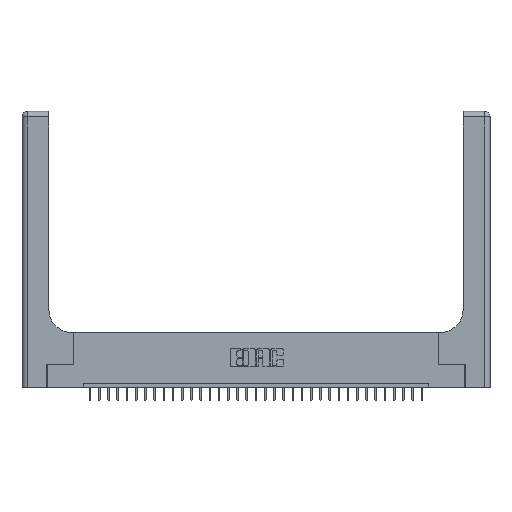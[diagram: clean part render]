
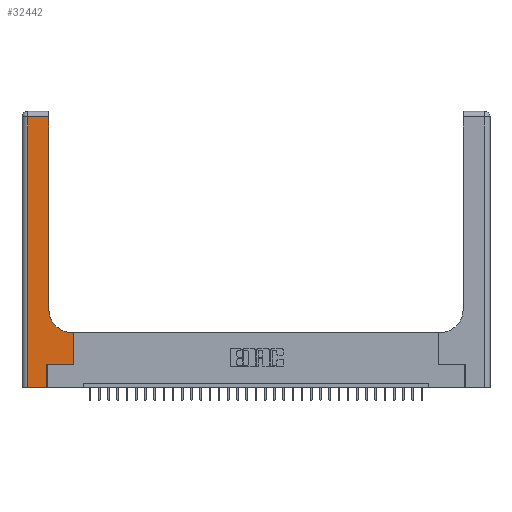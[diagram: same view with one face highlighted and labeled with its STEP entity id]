
A CAD part, top view. The second image highlights one B-rep face of the part: STEP entity #32442.
In plain terms, the highlighted planar face has unit normal (0, 0, 1).
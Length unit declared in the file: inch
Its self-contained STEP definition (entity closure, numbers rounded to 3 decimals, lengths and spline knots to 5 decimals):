
#429 = LINE ( 'NONE', #18204, #14327 ) ;
#706 = VECTOR ( 'NONE', #27612, 39.37008 ) ;
#1019 = ORIENTED_EDGE ( 'NONE', *, *, #8162, .T. ) ;
#1264 = CARTESIAN_POINT ( 'NONE',  ( 0., 3., 0.37 ) ) ;
#1698 = ORIENTED_EDGE ( 'NONE', *, *, #15949, .T. ) ;
#2231 = CARTESIAN_POINT ( 'NONE',  ( 0.2915, 2.94, 0.37 ) ) ;
#3149 = EDGE_CURVE ( 'NONE', #30729, #19124, #429, .T. ) ;
#3225 = CARTESIAN_POINT ( 'NONE',  ( 0.5585, 0.6, 0.37 ) ) ;
#3916 = VERTEX_POINT ( 'NONE', #15394 ) ;
#4030 = CARTESIAN_POINT ( 'NONE',  ( 0.5585, 0.25, 0.37 ) ) ;
#4856 = VERTEX_POINT ( 'NONE', #22774 ) ;
#4884 = VECTOR ( 'NONE', #11220, 39.37008 ) ;
#5099 = CARTESIAN_POINT ( 'NONE',  ( 0.269, 0.25, 0.37 ) ) ;
#5725 = VERTEX_POINT ( 'NONE', #14816 ) ;
#6224 = DIRECTION ( 'NONE',  ( 0., 0., -1. ) ) ;
#6456 = CARTESIAN_POINT ( 'NONE',  ( 0.269, 0.25, 0.37 ) ) ;
#6606 = AXIS2_PLACEMENT_3D ( 'NONE', #27712, #25154, #14715 ) ;
#7086 = EDGE_LOOP ( 'NONE', ( #30935, #1698, #17297, #32505, #23765, #1019, #29211, #14005, #7499 ) ) ;
#7499 = ORIENTED_EDGE ( 'NONE', *, *, #12055, .T. ) ;
#8162 = EDGE_CURVE ( 'NONE', #22408, #3916, #24742, .T. ) ;
#8231 = EDGE_CURVE ( 'NONE', #5725, #12000, #15760, .T. ) ;
#8516 = VERTEX_POINT ( 'NONE', #30452 ) ;
#8628 = AXIS2_PLACEMENT_3D ( 'NONE', #1264, #6224, #22279 ) ;
#9114 = CARTESIAN_POINT ( 'NONE',  ( 0., 0., 0.37 ) ) ;
#10355 = CARTESIAN_POINT ( 'NONE',  ( 0.269, 0., 0.37 ) ) ;
#11220 = DIRECTION ( 'NONE',  ( 1., 0., 0. ) ) ;
#12000 = VERTEX_POINT ( 'NONE', #2231 ) ;
#12055 = EDGE_CURVE ( 'NONE', #19124, #5725, #33334, .T. ) ;
#12588 = EDGE_CURVE ( 'NONE', #4856, #22408, #33799, .T. ) ;
#13820 = VECTOR ( 'NONE', #19882, 39.37008 ) ;
#13849 = CARTESIAN_POINT ( 'NONE',  ( 0.5415, 0.6, 0.37 ) ) ;
#14005 = ORIENTED_EDGE ( 'NONE', *, *, #3149, .T. ) ;
#14327 = VECTOR ( 'NONE', #21275, 39.37008 ) ;
#14525 = EDGE_CURVE ( 'NONE', #3916, #30729, #19733, .T. ) ;
#14715 = DIRECTION ( 'NONE',  ( 1., 0., 0. ) ) ;
#14816 = CARTESIAN_POINT ( 'NONE',  ( 0.2915, 0.85, 0.37 ) ) ;
#15394 = CARTESIAN_POINT ( 'NONE',  ( 0.5585, 0.25, 0.37 ) ) ;
#15760 = LINE ( 'NONE', #22509, #30517 ) ;
#15949 = EDGE_CURVE ( 'NONE', #12000, #8516, #23826, .T. ) ;
#15999 = CARTESIAN_POINT ( 'NONE',  ( 0.06, 0., 0.37 ) ) ;
#17297 = ORIENTED_EDGE ( 'NONE', *, *, #25033, .T. ) ;
#17875 = DIRECTION ( 'NONE',  ( 0., 1., 0. ) ) ;
#18204 = CARTESIAN_POINT ( 'NONE',  ( 0.2915, 0.6, 0.37 ) ) ;
#18245 = DIRECTION ( 'NONE',  ( 0., 1., 0. ) ) ;
#19029 = FACE_OUTER_BOUND ( 'NONE', #7086, .T. ) ;
#19124 = VERTEX_POINT ( 'NONE', #13849 ) ;
#19191 = CARTESIAN_POINT ( 'NONE',  ( 0., 2.94, 0.37 ) ) ;
#19733 = LINE ( 'NONE', #4030, #26926 ) ;
#19882 = DIRECTION ( 'NONE',  ( 1., 0., 0. ) ) ;
#19921 = LINE ( 'NONE', #32729, #706 ) ;
#21067 = VERTEX_POINT ( 'NONE', #15999 ) ;
#21275 = DIRECTION ( 'NONE',  ( -1., 0., 0. ) ) ;
#21936 = LINE ( 'NONE', #9114, #13820 ) ;
#22279 = DIRECTION ( 'NONE',  ( -1., 0., 0. ) ) ;
#22408 = VERTEX_POINT ( 'NONE', #5099 ) ;
#22509 = CARTESIAN_POINT ( 'NONE',  ( 0.2915, 3., 0.37 ) ) ;
#22774 = CARTESIAN_POINT ( 'NONE',  ( 0.269, 0., 0.37 ) ) ;
#23765 = ORIENTED_EDGE ( 'NONE', *, *, #12588, .T. ) ;
#23826 = LINE ( 'NONE', #19191, #32461 ) ;
#24644 = VECTOR ( 'NONE', #18245, 39.37008 ) ;
#24742 = LINE ( 'NONE', #6456, #4884 ) ;
#25033 = EDGE_CURVE ( 'NONE', #8516, #21067, #19921, .T. ) ;
#25154 = DIRECTION ( 'NONE',  ( 0., 0., -1. ) ) ;
#25566 = EDGE_CURVE ( 'NONE', #21067, #4856, #21936, .T. ) ;
#26901 = PLANE ( 'NONE',  #8628 ) ;
#26926 = VECTOR ( 'NONE', #30153, 39.37008 ) ;
#27612 = DIRECTION ( 'NONE',  ( 0., -1., 0. ) ) ;
#27712 = CARTESIAN_POINT ( 'NONE',  ( 0.5415, 0.85, 0.37 ) ) ;
#29211 = ORIENTED_EDGE ( 'NONE', *, *, #14525, .T. ) ;
#30153 = DIRECTION ( 'NONE',  ( 0., 1., 0. ) ) ;
#30452 = CARTESIAN_POINT ( 'NONE',  ( 0.06, 2.94, 0.37 ) ) ;
#30517 = VECTOR ( 'NONE', #17875, 39.37008 ) ;
#30729 = VERTEX_POINT ( 'NONE', #3225 ) ;
#30935 = ORIENTED_EDGE ( 'NONE', *, *, #8231, .T. ) ;
#31840 = DIRECTION ( 'NONE',  ( -1., 0., 0. ) ) ;
#32442 = ADVANCED_FACE ( 'NONE', ( #19029 ), #26901, .F. ) ;
#32461 = VECTOR ( 'NONE', #31840, 39.37008 ) ;
#32505 = ORIENTED_EDGE ( 'NONE', *, *, #25566, .T. ) ;
#32729 = CARTESIAN_POINT ( 'NONE',  ( 0.06, 3., 0.37 ) ) ;
#33334 = CIRCLE ( 'NONE', #6606, 0.25 ) ;
#33799 = LINE ( 'NONE', #10355, #24644 ) ;
